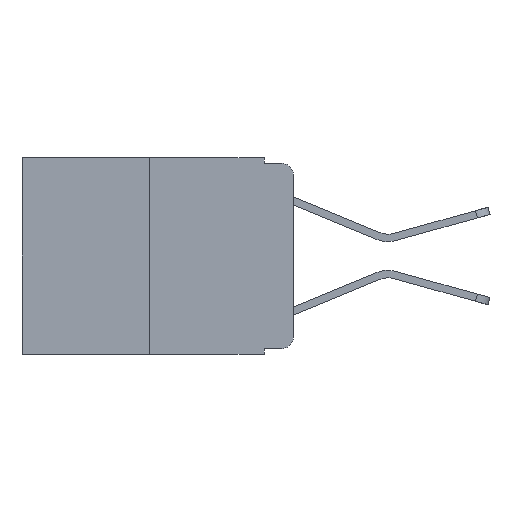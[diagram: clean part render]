
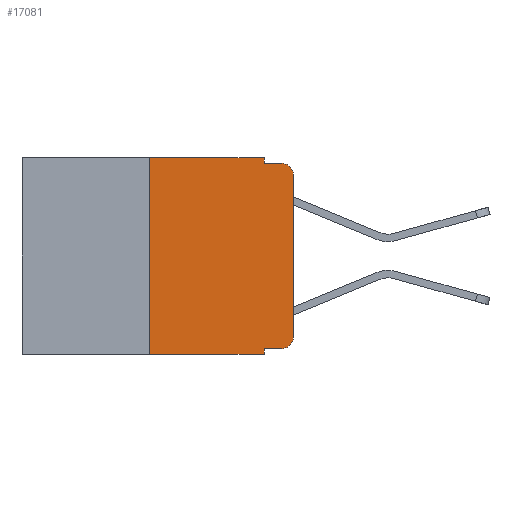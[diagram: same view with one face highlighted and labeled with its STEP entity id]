
A CAD part, left-side view. The second image highlights one B-rep face of the part: STEP entity #17081.
In plain terms, the highlighted planar face has unit normal (-1, 0, 0).
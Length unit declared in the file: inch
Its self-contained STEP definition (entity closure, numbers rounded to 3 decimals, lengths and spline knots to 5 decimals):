
#47 = EDGE_CURVE ( 'NONE', #9910, #8615, #3589, .T. ) ;
#228 = LINE ( 'NONE', #4857, #10590 ) ;
#715 = PLANE ( 'NONE',  #8749 ) ;
#725 = LINE ( 'NONE', #17484, #14800 ) ;
#1073 = VERTEX_POINT ( 'NONE', #16657 ) ;
#1079 = EDGE_CURVE ( 'NONE', #9910, #16030, #5556, .T. ) ;
#1427 = DIRECTION ( 'NONE',  ( 0., 0., 1. ) ) ;
#1645 = CARTESIAN_POINT ( 'NONE',  ( 0., 0.02, -0.03 ) ) ;
#1822 = ORIENTED_EDGE ( 'NONE', *, *, #3070, .F. ) ;
#1840 = LINE ( 'NONE', #15732, #6111 ) ;
#1956 = CIRCLE ( 'NONE', #8179, 0.02 ) ;
#2091 = EDGE_CURVE ( 'NONE', #9798, #1073, #12556, .T. ) ;
#2234 = DIRECTION ( 'NONE',  ( 0., 0., -1. ) ) ;
#2292 = ORIENTED_EDGE ( 'NONE', *, *, #2091, .F. ) ;
#2526 = CIRCLE ( 'NONE', #8212, 0.02 ) ;
#2744 = ORIENTED_EDGE ( 'NONE', *, *, #47, .T. ) ;
#3070 = EDGE_CURVE ( 'NONE', #9608, #11841, #4379, .T. ) ;
#3139 = DIRECTION ( 'NONE',  ( 0., 0., -1. ) ) ;
#3589 = LINE ( 'NONE', #9773, #17226 ) ;
#4066 = EDGE_CURVE ( 'NONE', #11841, #5585, #9555, .T. ) ;
#4379 = LINE ( 'NONE', #4522, #5257 ) ;
#4522 = CARTESIAN_POINT ( 'NONE',  ( 0., 0.051, 0. ) ) ;
#4857 = CARTESIAN_POINT ( 'NONE',  ( 0., 0.473, -0.343 ) ) ;
#5017 = EDGE_CURVE ( 'NONE', #13439, #5585, #1956, .T. ) ;
#5257 = VECTOR ( 'NONE', #15157, 39.37008 ) ;
#5276 = DIRECTION ( 'NONE',  ( 0., -1., 0. ) ) ;
#5556 = LINE ( 'NONE', #16605, #15230 ) ;
#5585 = VERTEX_POINT ( 'NONE', #7616 ) ;
#5761 = CARTESIAN_POINT ( 'NONE',  ( 0., 0.02, -0.313 ) ) ;
#5943 = EDGE_CURVE ( 'NONE', #8801, #13439, #725, .T. ) ;
#6097 = ORIENTED_EDGE ( 'NONE', *, *, #12233, .T. ) ;
#6111 = VECTOR ( 'NONE', #5276, 39.37008 ) ;
#6354 = VECTOR ( 'NONE', #13308, 39.37008 ) ;
#6715 = EDGE_LOOP ( 'NONE', ( #8497, #15342, #15722, #1822, #12720, #2292, #6097, #9715, #2744, #10140 ) ) ;
#7156 = DIRECTION ( 'NONE',  ( 0., -1., 0. ) ) ;
#7161 = DIRECTION ( 'NONE',  ( 0., 0., -1. ) ) ;
#7515 = CARTESIAN_POINT ( 'NONE',  ( 0., 0.051, -0.333 ) ) ;
#7616 = CARTESIAN_POINT ( 'NONE',  ( 0., 0.02, -0.01 ) ) ;
#8179 = AXIS2_PLACEMENT_3D ( 'NONE', #1645, #11327, #3139 ) ;
#8212 = AXIS2_PLACEMENT_3D ( 'NONE', #5761, #14948, #7161 ) ;
#8329 = CARTESIAN_POINT ( 'NONE',  ( 0., 0.051, -0.01 ) ) ;
#8497 = ORIENTED_EDGE ( 'NONE', *, *, #5943, .T. ) ;
#8615 = VERTEX_POINT ( 'NONE', #14893 ) ;
#8749 = AXIS2_PLACEMENT_3D ( 'NONE', #9236, #10529, #2234 ) ;
#8801 = VERTEX_POINT ( 'NONE', #16437 ) ;
#9236 = CARTESIAN_POINT ( 'NONE',  ( 0., 0.473, 0. ) ) ;
#9555 = LINE ( 'NONE', #8329, #11514 ) ;
#9608 = VERTEX_POINT ( 'NONE', #15537 ) ;
#9715 = ORIENTED_EDGE ( 'NONE', *, *, #1079, .F. ) ;
#9773 = CARTESIAN_POINT ( 'NONE',  ( 0., 0.051, -0.333 ) ) ;
#9798 = VERTEX_POINT ( 'NONE', #9958 ) ;
#9910 = VERTEX_POINT ( 'NONE', #7515 ) ;
#9937 = CARTESIAN_POINT ( 'NONE',  ( 0., 0.051, -0.343 ) ) ;
#9958 = CARTESIAN_POINT ( 'NONE',  ( 0., 0.25, -0.343 ) ) ;
#10140 = ORIENTED_EDGE ( 'NONE', *, *, #16758, .T. ) ;
#10284 = DIRECTION ( 'NONE',  ( 0., -1., 0. ) ) ;
#10529 = DIRECTION ( 'NONE',  ( 1., 0., 0. ) ) ;
#10590 = VECTOR ( 'NONE', #10284, 39.37008 ) ;
#11005 = CARTESIAN_POINT ( 'NONE',  ( 0., 0.051, -0.01 ) ) ;
#11327 = DIRECTION ( 'NONE',  ( -1., 0., 0. ) ) ;
#11514 = VECTOR ( 'NONE', #16067, 39.37008 ) ;
#11841 = VERTEX_POINT ( 'NONE', #11005 ) ;
#12233 = EDGE_CURVE ( 'NONE', #9798, #16030, #228, .T. ) ;
#12556 = LINE ( 'NONE', #17441, #6354 ) ;
#12720 = ORIENTED_EDGE ( 'NONE', *, *, #16475, .F. ) ;
#13104 = FACE_OUTER_BOUND ( 'NONE', #6715, .T. ) ;
#13308 = DIRECTION ( 'NONE',  ( 0., 0., 1. ) ) ;
#13439 = VERTEX_POINT ( 'NONE', #15656 ) ;
#14800 = VECTOR ( 'NONE', #1427, 39.37008 ) ;
#14893 = CARTESIAN_POINT ( 'NONE',  ( 0., 0.02, -0.333 ) ) ;
#14948 = DIRECTION ( 'NONE',  ( -1., 0., 0. ) ) ;
#15157 = DIRECTION ( 'NONE',  ( 0., 0., -1. ) ) ;
#15230 = VECTOR ( 'NONE', #16517, 39.37008 ) ;
#15342 = ORIENTED_EDGE ( 'NONE', *, *, #5017, .T. ) ;
#15537 = CARTESIAN_POINT ( 'NONE',  ( 0., 0.051, 0. ) ) ;
#15656 = CARTESIAN_POINT ( 'NONE',  ( 0., 0., -0.03 ) ) ;
#15722 = ORIENTED_EDGE ( 'NONE', *, *, #4066, .F. ) ;
#15732 = CARTESIAN_POINT ( 'NONE',  ( 0., 0.473, 0. ) ) ;
#16030 = VERTEX_POINT ( 'NONE', #9937 ) ;
#16067 = DIRECTION ( 'NONE',  ( 0., -1., 0. ) ) ;
#16437 = CARTESIAN_POINT ( 'NONE',  ( 0., 0., -0.313 ) ) ;
#16475 = EDGE_CURVE ( 'NONE', #1073, #9608, #1840, .T. ) ;
#16517 = DIRECTION ( 'NONE',  ( 0., 0., -1. ) ) ;
#16605 = CARTESIAN_POINT ( 'NONE',  ( 0., 0.051, 0. ) ) ;
#16657 = CARTESIAN_POINT ( 'NONE',  ( 0., 0.25, 0. ) ) ;
#16758 = EDGE_CURVE ( 'NONE', #8615, #8801, #2526, .T. ) ;
#17081 = ADVANCED_FACE ( 'NONE', ( #13104 ), #715, .F. ) ;
#17226 = VECTOR ( 'NONE', #7156, 39.37008 ) ;
#17441 = CARTESIAN_POINT ( 'NONE',  ( 0., 0.25, 0. ) ) ;
#17484 = CARTESIAN_POINT ( 'NONE',  ( 0., 0., 0. ) ) ;
